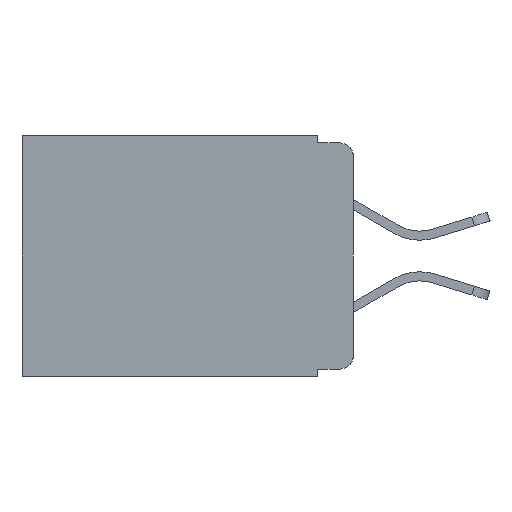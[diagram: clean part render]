
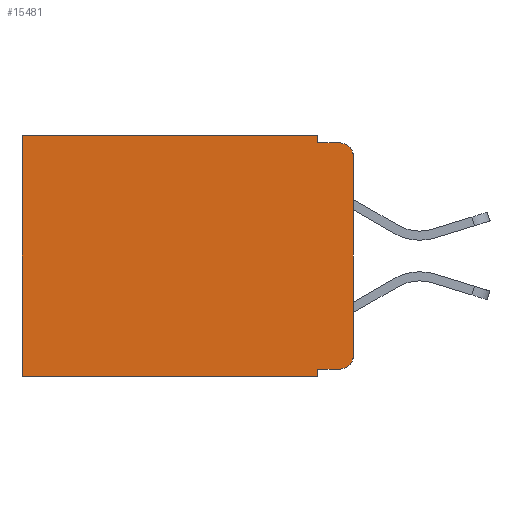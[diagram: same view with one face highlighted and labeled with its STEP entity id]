
A CAD part, left-side view. The second image highlights one B-rep face of the part: STEP entity #15481.
In plain terms, the highlighted planar face has unit normal (-1, 0, 0).
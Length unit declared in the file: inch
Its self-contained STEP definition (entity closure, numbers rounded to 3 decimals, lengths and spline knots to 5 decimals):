
#893 = CARTESIAN_POINT ( 'NONE',  ( 0.298, 0., 0. ) ) ;
#925 = VERTEX_POINT ( 'NONE', #10659 ) ;
#1059 = CARTESIAN_POINT ( 'NONE',  ( 0.298, 0.473, -0.343 ) ) ;
#1198 = AXIS2_PLACEMENT_3D ( 'NONE', #17861, #17795, #16175 ) ;
#1202 = ORIENTED_EDGE ( 'NONE', *, *, #4200, .F. ) ;
#1221 = EDGE_CURVE ( 'NONE', #12058, #11269, #10473, .T. ) ;
#1469 = VECTOR ( 'NONE', #12656, 39.37008 ) ;
#2069 = VERTEX_POINT ( 'NONE', #13615 ) ;
#2283 = ORIENTED_EDGE ( 'NONE', *, *, #13247, .T. ) ;
#2356 = VECTOR ( 'NONE', #6203, 39.37008 ) ;
#2750 = DIRECTION ( 'NONE',  ( 0., 1., 0. ) ) ;
#2770 = CARTESIAN_POINT ( 'NONE',  ( 0.298, 0.051, -0.01 ) ) ;
#3230 = ORIENTED_EDGE ( 'NONE', *, *, #5230, .F. ) ;
#3621 = ORIENTED_EDGE ( 'NONE', *, *, #4707, .F. ) ;
#3724 = VECTOR ( 'NONE', #10021, 39.37008 ) ;
#4159 = DIRECTION ( 'NONE',  ( 0., 1., 0. ) ) ;
#4200 = EDGE_CURVE ( 'NONE', #15988, #925, #18562, .T. ) ;
#4600 = EDGE_LOOP ( 'NONE', ( #3621, #20689, #11282, #3230, #14628, #5718, #7025, #1202, #14591, #2283 ) ) ;
#4707 = EDGE_CURVE ( 'NONE', #12058, #19854, #5760, .T. ) ;
#4937 = FACE_OUTER_BOUND ( 'NONE', #4600, .T. ) ;
#5230 = EDGE_CURVE ( 'NONE', #8694, #2069, #21085, .T. ) ;
#5459 = CARTESIAN_POINT ( 'NONE',  ( 0.298, 0.02, -0.01 ) ) ;
#5718 = ORIENTED_EDGE ( 'NONE', *, *, #10806, .T. ) ;
#5760 = LINE ( 'NONE', #17595, #1469 ) ;
#5952 = CARTESIAN_POINT ( 'NONE',  ( 0.298, 0., -0.343 ) ) ;
#5973 = LINE ( 'NONE', #6778, #13361 ) ;
#6203 = DIRECTION ( 'NONE',  ( 0., 0., -1. ) ) ;
#6766 = EDGE_CURVE ( 'NONE', #8694, #15832, #20390, .T. ) ;
#6778 = CARTESIAN_POINT ( 'NONE',  ( 0.298, 0.051, -0.333 ) ) ;
#7025 = ORIENTED_EDGE ( 'NONE', *, *, #15864, .F. ) ;
#7143 = CARTESIAN_POINT ( 'NONE',  ( 0.298, 0.02, -0.313 ) ) ;
#7852 = CARTESIAN_POINT ( 'NONE',  ( 0.298, 0.473, 0. ) ) ;
#7960 = CARTESIAN_POINT ( 'NONE',  ( 0.298, 0.051, -0.333 ) ) ;
#8124 = AXIS2_PLACEMENT_3D ( 'NONE', #16833, #18441, #13442 ) ;
#8694 = VERTEX_POINT ( 'NONE', #14494 ) ;
#8746 = CARTESIAN_POINT ( 'NONE',  ( 0.298, 0., -0.03 ) ) ;
#9851 = VECTOR ( 'NONE', #20105, 39.37008 ) ;
#10019 = DIRECTION ( 'NONE',  ( 0., -1., 0. ) ) ;
#10021 = DIRECTION ( 'NONE',  ( 0., 0., -1. ) ) ;
#10227 = LINE ( 'NONE', #7852, #2356 ) ;
#10473 = CIRCLE ( 'NONE', #1198, 0.02 ) ;
#10659 = CARTESIAN_POINT ( 'NONE',  ( 0.298, 0.051, -0.343 ) ) ;
#10806 = EDGE_CURVE ( 'NONE', #15832, #14073, #10227, .T. ) ;
#11269 = VERTEX_POINT ( 'NONE', #5459 ) ;
#11282 = ORIENTED_EDGE ( 'NONE', *, *, #19689, .F. ) ;
#11674 = LINE ( 'NONE', #2770, #19845 ) ;
#12058 = VERTEX_POINT ( 'NONE', #8746 ) ;
#12419 = CARTESIAN_POINT ( 'NONE',  ( 0.298, 0.02, -0.333 ) ) ;
#12656 = DIRECTION ( 'NONE',  ( 0., 0., -1. ) ) ;
#12868 = AXIS2_PLACEMENT_3D ( 'NONE', #7143, #20543, #19095 ) ;
#13247 = EDGE_CURVE ( 'NONE', #19341, #19854, #13689, .T. ) ;
#13361 = VECTOR ( 'NONE', #10019, 39.37008 ) ;
#13442 = DIRECTION ( 'NONE',  ( 0., 0., -1. ) ) ;
#13472 = CARTESIAN_POINT ( 'NONE',  ( 0.298, 0.051, 0. ) ) ;
#13615 = CARTESIAN_POINT ( 'NONE',  ( 0.298, 0.051, -0.01 ) ) ;
#13689 = CIRCLE ( 'NONE', #12868, 0.02 ) ;
#14015 = VECTOR ( 'NONE', #4159, 39.37008 ) ;
#14073 = VERTEX_POINT ( 'NONE', #1059 ) ;
#14399 = DIRECTION ( 'NONE',  ( 0., -1., 0. ) ) ;
#14494 = CARTESIAN_POINT ( 'NONE',  ( 0.298, 0.051, 0. ) ) ;
#14591 = ORIENTED_EDGE ( 'NONE', *, *, #14996, .T. ) ;
#14628 = ORIENTED_EDGE ( 'NONE', *, *, #6766, .T. ) ;
#14668 = CARTESIAN_POINT ( 'NONE',  ( 0.298, 0., -0.313 ) ) ;
#14854 = LINE ( 'NONE', #5952, #15642 ) ;
#14996 = EDGE_CURVE ( 'NONE', #15988, #19341, #5973, .T. ) ;
#15481 = ADVANCED_FACE ( 'NONE', ( #4937 ), #19800, .F. ) ;
#15586 = CARTESIAN_POINT ( 'NONE',  ( 0.298, 0.473, 0. ) ) ;
#15642 = VECTOR ( 'NONE', #2750, 39.37008 ) ;
#15832 = VERTEX_POINT ( 'NONE', #15586 ) ;
#15864 = EDGE_CURVE ( 'NONE', #925, #14073, #14854, .T. ) ;
#15988 = VERTEX_POINT ( 'NONE', #7960 ) ;
#16175 = DIRECTION ( 'NONE',  ( 0., 0., -1. ) ) ;
#16572 = CARTESIAN_POINT ( 'NONE',  ( 0.298, 0.051, 0. ) ) ;
#16833 = CARTESIAN_POINT ( 'NONE',  ( 0.298, 0., 0. ) ) ;
#17595 = CARTESIAN_POINT ( 'NONE',  ( 0.298, 0., 0. ) ) ;
#17795 = DIRECTION ( 'NONE',  ( -1., 0., 0. ) ) ;
#17861 = CARTESIAN_POINT ( 'NONE',  ( 0.298, 0.02, -0.03 ) ) ;
#18441 = DIRECTION ( 'NONE',  ( 1., 0., 0. ) ) ;
#18562 = LINE ( 'NONE', #13472, #9851 ) ;
#19095 = DIRECTION ( 'NONE',  ( 0., 0., -1. ) ) ;
#19341 = VERTEX_POINT ( 'NONE', #12419 ) ;
#19689 = EDGE_CURVE ( 'NONE', #2069, #11269, #11674, .T. ) ;
#19800 = PLANE ( 'NONE',  #8124 ) ;
#19845 = VECTOR ( 'NONE', #14399, 39.37008 ) ;
#19854 = VERTEX_POINT ( 'NONE', #14668 ) ;
#20105 = DIRECTION ( 'NONE',  ( 0., 0., -1. ) ) ;
#20390 = LINE ( 'NONE', #893, #14015 ) ;
#20543 = DIRECTION ( 'NONE',  ( -1., 0., 0. ) ) ;
#20689 = ORIENTED_EDGE ( 'NONE', *, *, #1221, .T. ) ;
#21085 = LINE ( 'NONE', #16572, #3724 ) ;
